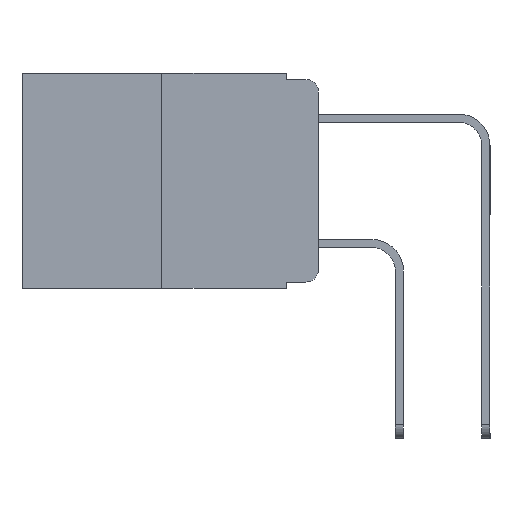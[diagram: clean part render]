
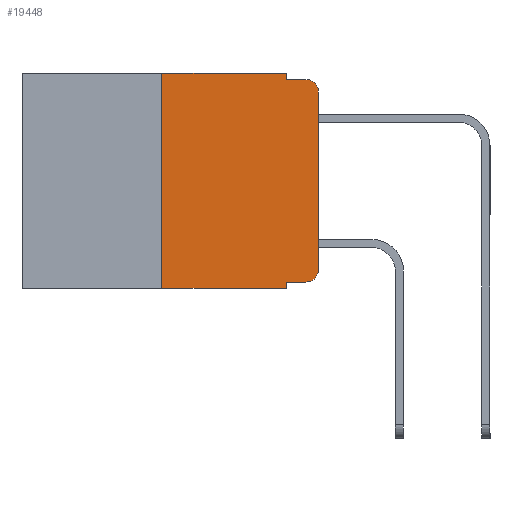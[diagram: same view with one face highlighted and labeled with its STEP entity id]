
A CAD part, left-side view. The second image highlights one B-rep face of the part: STEP entity #19448.
In plain terms, the highlighted planar face has unit normal (-1, 0, 0).
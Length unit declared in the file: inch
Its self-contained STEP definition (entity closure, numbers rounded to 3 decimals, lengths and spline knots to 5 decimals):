
#28 = CIRCLE ( 'NONE', #4532, 0.02 ) ;
#697 = CARTESIAN_POINT ( 'NONE',  ( 0., 0.02, -0.01 ) ) ;
#721 = DIRECTION ( 'NONE',  ( 0., -1., 0. ) ) ;
#971 = DIRECTION ( 'NONE',  ( 0., 0., 1. ) ) ;
#1157 = VECTOR ( 'NONE', #5268, 39.37008 ) ;
#1355 = PLANE ( 'NONE',  #8692 ) ;
#1461 = CARTESIAN_POINT ( 'NONE',  ( 0., 0.02, -0.313 ) ) ;
#2010 = VERTEX_POINT ( 'NONE', #15262 ) ;
#2140 = CARTESIAN_POINT ( 'NONE',  ( 0., 0.25, 0. ) ) ;
#2550 = CARTESIAN_POINT ( 'NONE',  ( 0., 0.02, -0.333 ) ) ;
#2735 = CARTESIAN_POINT ( 'NONE',  ( 0., 0.051, -0.343 ) ) ;
#3092 = VERTEX_POINT ( 'NONE', #19360 ) ;
#3228 = DIRECTION ( 'NONE',  ( 0., 0., -1. ) ) ;
#3436 = LINE ( 'NONE', #15222, #20484 ) ;
#3535 = CARTESIAN_POINT ( 'NONE',  ( 0., 0.473, -0.343 ) ) ;
#3611 = VECTOR ( 'NONE', #17692, 39.37008 ) ;
#3967 = CARTESIAN_POINT ( 'NONE',  ( 0., 0.051, 0. ) ) ;
#4139 = CARTESIAN_POINT ( 'NONE',  ( 0., 0.051, -0.333 ) ) ;
#4248 = EDGE_LOOP ( 'NONE', ( #9502, #16953, #8494, #19617, #10688, #20248, #6762, #5371, #11327, #8183 ) ) ;
#4532 = AXIS2_PLACEMENT_3D ( 'NONE', #18971, #9259, #20534 ) ;
#4828 = DIRECTION ( 'NONE',  ( 1., 0., 0. ) ) ;
#4998 = EDGE_CURVE ( 'NONE', #3092, #8347, #7590, .T. ) ;
#5268 = DIRECTION ( 'NONE',  ( 0., -1., 0. ) ) ;
#5371 = ORIENTED_EDGE ( 'NONE', *, *, #6166, .F. ) ;
#6166 = EDGE_CURVE ( 'NONE', #13869, #15894, #3436, .T. ) ;
#6353 = VERTEX_POINT ( 'NONE', #697 ) ;
#6376 = AXIS2_PLACEMENT_3D ( 'NONE', #1461, #13406, #3228 ) ;
#6762 = ORIENTED_EDGE ( 'NONE', *, *, #8825, .T. ) ;
#6927 = LINE ( 'NONE', #19279, #19491 ) ;
#7020 = DIRECTION ( 'NONE',  ( 0., 0., -1. ) ) ;
#7351 = EDGE_CURVE ( 'NONE', #13869, #20709, #11970, .T. ) ;
#7512 = CIRCLE ( 'NONE', #6376, 0.02 ) ;
#7590 = LINE ( 'NONE', #16724, #19576 ) ;
#8051 = VERTEX_POINT ( 'NONE', #8135 ) ;
#8135 = CARTESIAN_POINT ( 'NONE',  ( 0., 0.051, 0. ) ) ;
#8183 = ORIENTED_EDGE ( 'NONE', *, *, #10755, .T. ) ;
#8347 = VERTEX_POINT ( 'NONE', #2140 ) ;
#8494 = ORIENTED_EDGE ( 'NONE', *, *, #8519, .F. ) ;
#8519 = EDGE_CURVE ( 'NONE', #2010, #6353, #12741, .T. ) ;
#8692 = AXIS2_PLACEMENT_3D ( 'NONE', #14884, #4828, #16502 ) ;
#8825 = EDGE_CURVE ( 'NONE', #3092, #15894, #10334, .T. ) ;
#9259 = DIRECTION ( 'NONE',  ( -1., 0., 0. ) ) ;
#9341 = CARTESIAN_POINT ( 'NONE',  ( 0., 0., -0.313 ) ) ;
#9502 = ORIENTED_EDGE ( 'NONE', *, *, #11905, .T. ) ;
#9656 = EDGE_CURVE ( 'NONE', #8051, #2010, #18638, .T. ) ;
#9887 = CARTESIAN_POINT ( 'NONE',  ( 0., 0.051, -0.333 ) ) ;
#10043 = VECTOR ( 'NONE', #14179, 39.37008 ) ;
#10334 = LINE ( 'NONE', #3535, #1157 ) ;
#10688 = ORIENTED_EDGE ( 'NONE', *, *, #16746, .F. ) ;
#10755 = EDGE_CURVE ( 'NONE', #20709, #20654, #7512, .T. ) ;
#11327 = ORIENTED_EDGE ( 'NONE', *, *, #7351, .T. ) ;
#11905 = EDGE_CURVE ( 'NONE', #20654, #19507, #6927, .T. ) ;
#11910 = DIRECTION ( 'NONE',  ( 0., -1., 0. ) ) ;
#11970 = LINE ( 'NONE', #4139, #15726 ) ;
#12741 = LINE ( 'NONE', #14558, #3611 ) ;
#13031 = EDGE_CURVE ( 'NONE', #19507, #6353, #28, .T. ) ;
#13406 = DIRECTION ( 'NONE',  ( -1., 0., 0. ) ) ;
#13869 = VERTEX_POINT ( 'NONE', #9887 ) ;
#14179 = DIRECTION ( 'NONE',  ( 0., 0., -1. ) ) ;
#14558 = CARTESIAN_POINT ( 'NONE',  ( 0., 0.051, -0.01 ) ) ;
#14811 = LINE ( 'NONE', #19802, #18555 ) ;
#14884 = CARTESIAN_POINT ( 'NONE',  ( 0., 0.473, 0. ) ) ;
#15222 = CARTESIAN_POINT ( 'NONE',  ( 0., 0.051, 0. ) ) ;
#15262 = CARTESIAN_POINT ( 'NONE',  ( 0., 0.051, -0.01 ) ) ;
#15726 = VECTOR ( 'NONE', #721, 39.37008 ) ;
#15894 = VERTEX_POINT ( 'NONE', #2735 ) ;
#16502 = DIRECTION ( 'NONE',  ( 0., 0., -1. ) ) ;
#16724 = CARTESIAN_POINT ( 'NONE',  ( 0., 0.25, 0. ) ) ;
#16746 = EDGE_CURVE ( 'NONE', #8347, #8051, #14811, .T. ) ;
#16770 = DIRECTION ( 'NONE',  ( 0., 0., 1. ) ) ;
#16951 = FACE_OUTER_BOUND ( 'NONE', #4248, .T. ) ;
#16953 = ORIENTED_EDGE ( 'NONE', *, *, #13031, .T. ) ;
#17692 = DIRECTION ( 'NONE',  ( 0., -1., 0. ) ) ;
#18555 = VECTOR ( 'NONE', #11910, 39.37008 ) ;
#18638 = LINE ( 'NONE', #3967, #10043 ) ;
#18971 = CARTESIAN_POINT ( 'NONE',  ( 0., 0.02, -0.03 ) ) ;
#19279 = CARTESIAN_POINT ( 'NONE',  ( 0., 0., 0. ) ) ;
#19360 = CARTESIAN_POINT ( 'NONE',  ( 0., 0.25, -0.343 ) ) ;
#19448 = ADVANCED_FACE ( 'NONE', ( #16951 ), #1355, .F. ) ;
#19491 = VECTOR ( 'NONE', #971, 39.37008 ) ;
#19507 = VERTEX_POINT ( 'NONE', #21287 ) ;
#19576 = VECTOR ( 'NONE', #16770, 39.37008 ) ;
#19617 = ORIENTED_EDGE ( 'NONE', *, *, #9656, .F. ) ;
#19802 = CARTESIAN_POINT ( 'NONE',  ( 0., 0.473, 0. ) ) ;
#20248 = ORIENTED_EDGE ( 'NONE', *, *, #4998, .F. ) ;
#20484 = VECTOR ( 'NONE', #7020, 39.37008 ) ;
#20534 = DIRECTION ( 'NONE',  ( 0., 0., -1. ) ) ;
#20654 = VERTEX_POINT ( 'NONE', #9341 ) ;
#20709 = VERTEX_POINT ( 'NONE', #2550 ) ;
#21287 = CARTESIAN_POINT ( 'NONE',  ( 0., 0., -0.03 ) ) ;
